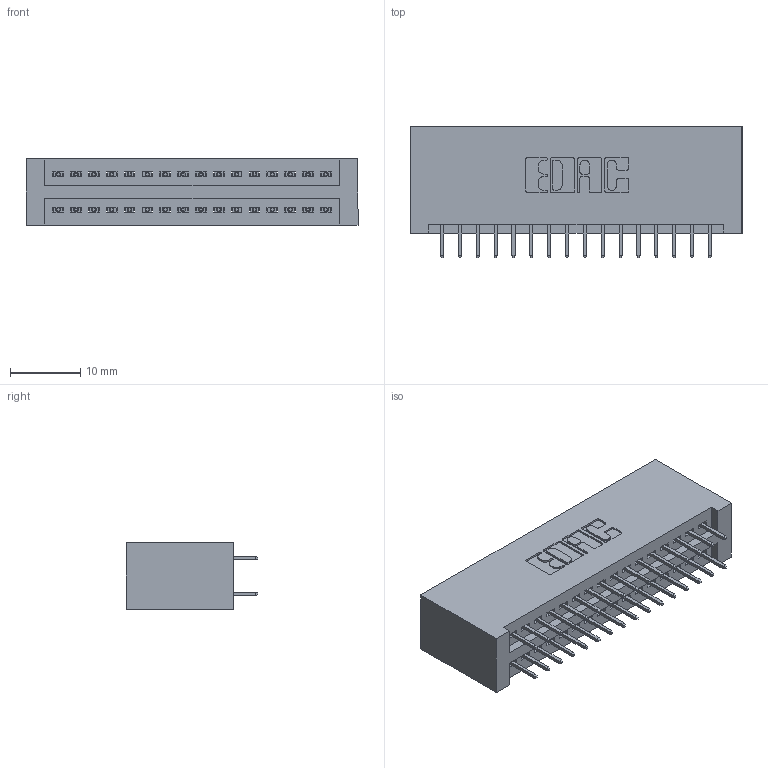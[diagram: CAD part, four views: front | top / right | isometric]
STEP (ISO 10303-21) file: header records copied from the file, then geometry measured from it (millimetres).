
FILE_DESCRIPTION (( 'STEP AP203' ), '1' );
FILE_NAME ('395-032-525-201.STEP', '2020-09-23T20:53:17', ( '' ), ( '' ), 'SwSTEP 2.0', 'SolidWorks 2020', '' );
FILE_SCHEMA (( 'CONFIG_CONTROL_DESIGN' ));
Length unit declared in the file: inch
Products named in the file (3): 395-032-525-201; 345 Part_No Mounting Lugs; 345-292-001_345-293-125
Assembly tree (33 placements, depth 2):
  395-032-525-201
    345 Part_No Mounting Lugs
    345-292-001_345-293-125  x32
Bounding box: 47.24 x 18.72 x 9.4 mm (x, y, z)
Volume: 4911.2 mm3; surface area: 6900.6 mm2
Topology: 33 solids, 33 shells, 1846 faces, 5213 edges, 3346 vertices
Faces by surface type: plane 1324, cylinder 522
Entity records: 15851 total; most frequent: CARTESIAN_POINT 2680, ORIENTED_EDGE 2614, DIRECTION 2391, EDGE_CURVE 1307, LINE 1123, VECTOR 1123, VERTEX_POINT 866, AXIS2_PLACEMENT_3D 634
